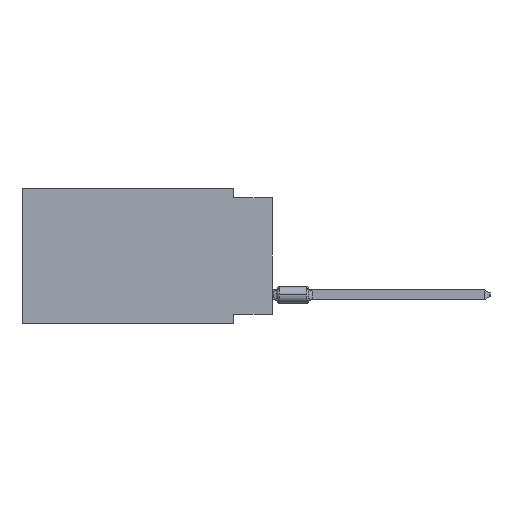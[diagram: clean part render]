
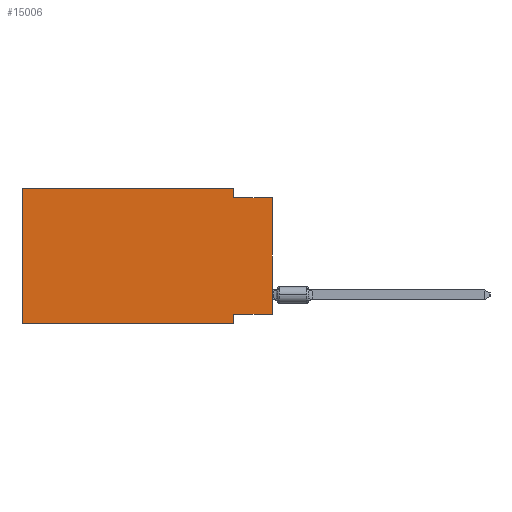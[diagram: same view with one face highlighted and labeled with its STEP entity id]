
A CAD part, left-side view. The second image highlights one B-rep face of the part: STEP entity #15006.
In plain terms, the highlighted planar face has unit normal (-1, 0, 0).
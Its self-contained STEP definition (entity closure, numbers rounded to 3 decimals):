
#209 = VERTEX_POINT ( 'NONE', #43237 ) ;
#4136 = EDGE_LOOP ( 'NONE', ( #37250, #56222, #58928, #13688, #12951, #16523, #34492, #6869 ) ) ;
#4829 = DIRECTION ( 'NONE',  ( 0., -1., 0. ) ) ;
#5136 = CARTESIAN_POINT ( 'NONE',  ( 0., 0., -0.635 ) ) ;
#6869 = ORIENTED_EDGE ( 'NONE', *, *, #29010, .F. ) ;
#7972 = LINE ( 'NONE', #22600, #20608 ) ;
#8087 = DIRECTION ( 'NONE',  ( 0., 0., -1. ) ) ;
#8434 = DIRECTION ( 'NONE',  ( 0., 0., 1. ) ) ;
#9926 = LINE ( 'NONE', #5136, #43193 ) ;
#11320 = CARTESIAN_POINT ( 'NONE',  ( 0., 16.383, 0. ) ) ;
#11420 = EDGE_CURVE ( 'NONE', #49928, #30665, #17992, .T. ) ;
#12259 = DIRECTION ( 'NONE',  ( 0., 0., -1. ) ) ;
#12860 = DIRECTION ( 'NONE',  ( 1., 0., 0. ) ) ;
#12913 = VERTEX_POINT ( 'NONE', #36321 ) ;
#12951 = ORIENTED_EDGE ( 'NONE', *, *, #53997, .F. ) ;
#13688 = ORIENTED_EDGE ( 'NONE', *, *, #23659, .F. ) ;
#15006 = ADVANCED_FACE ( 'NONE', ( #26875 ), #35800, .F. ) ;
#15818 = VERTEX_POINT ( 'NONE', #46158 ) ;
#16523 = ORIENTED_EDGE ( 'NONE', *, *, #24116, .T. ) ;
#17992 = LINE ( 'NONE', #62234, #51945 ) ;
#18377 = LINE ( 'NONE', #28557, #27778 ) ;
#19255 = VECTOR ( 'NONE', #44819, 1000. ) ;
#19465 = CARTESIAN_POINT ( 'NONE',  ( 0., 0., -8.255 ) ) ;
#20072 = CARTESIAN_POINT ( 'NONE',  ( 0., 16.383, 0. ) ) ;
#20608 = VECTOR ( 'NONE', #42022, 1000. ) ;
#22600 = CARTESIAN_POINT ( 'NONE',  ( 0., 16.383, 0. ) ) ;
#23659 = EDGE_CURVE ( 'NONE', #49332, #15818, #7972, .T. ) ;
#24116 = EDGE_CURVE ( 'NONE', #209, #12913, #18377, .T. ) ;
#24132 = VECTOR ( 'NONE', #63009, 1000. ) ;
#24517 = LINE ( 'NONE', #20072, #24132 ) ;
#26875 = FACE_OUTER_BOUND ( 'NONE', #4136, .T. ) ;
#27033 = LINE ( 'NONE', #41981, #29446 ) ;
#27778 = VECTOR ( 'NONE', #53075, 1000. ) ;
#28557 = CARTESIAN_POINT ( 'NONE',  ( 0., 16.383, -8.89 ) ) ;
#29010 = EDGE_CURVE ( 'NONE', #49928, #47721, #27033, .T. ) ;
#29446 = VECTOR ( 'NONE', #61087, 1000. ) ;
#30665 = VERTEX_POINT ( 'NONE', #57943 ) ;
#34492 = ORIENTED_EDGE ( 'NONE', *, *, #48266, .F. ) ;
#35800 = PLANE ( 'NONE',  #53589 ) ;
#36321 = CARTESIAN_POINT ( 'NONE',  ( 0., 2.54, -8.89 ) ) ;
#37250 = ORIENTED_EDGE ( 'NONE', *, *, #11420, .T. ) ;
#37402 = CARTESIAN_POINT ( 'NONE',  ( 0., 2.54, 0. ) ) ;
#41237 = LINE ( 'NONE', #37402, #59203 ) ;
#41981 = CARTESIAN_POINT ( 'NONE',  ( 0., 0., -8.255 ) ) ;
#42022 = DIRECTION ( 'NONE',  ( 0., -1., 0. ) ) ;
#43193 = VECTOR ( 'NONE', #4829, 1000. ) ;
#43237 = CARTESIAN_POINT ( 'NONE',  ( 0., 16.383, -8.89 ) ) ;
#43377 = EDGE_CURVE ( 'NONE', #49168, #30665, #9926, .T. ) ;
#44511 = LINE ( 'NONE', #49907, #19255 ) ;
#44819 = DIRECTION ( 'NONE',  ( 0., 0., -1. ) ) ;
#45372 = CARTESIAN_POINT ( 'NONE',  ( 0., 16.383, 0. ) ) ;
#45767 = EDGE_CURVE ( 'NONE', #15818, #49168, #41237, .T. ) ;
#46158 = CARTESIAN_POINT ( 'NONE',  ( 0., 2.54, 0. ) ) ;
#47721 = VERTEX_POINT ( 'NONE', #61026 ) ;
#48266 = EDGE_CURVE ( 'NONE', #47721, #12913, #44511, .T. ) ;
#49168 = VERTEX_POINT ( 'NONE', #53375 ) ;
#49332 = VERTEX_POINT ( 'NONE', #11320 ) ;
#49907 = CARTESIAN_POINT ( 'NONE',  ( 0., 2.54, -8.89 ) ) ;
#49928 = VERTEX_POINT ( 'NONE', #19465 ) ;
#51945 = VECTOR ( 'NONE', #8434, 1000. ) ;
#53075 = DIRECTION ( 'NONE',  ( 0., -1., 0. ) ) ;
#53375 = CARTESIAN_POINT ( 'NONE',  ( 0., 2.54, -0.635 ) ) ;
#53589 = AXIS2_PLACEMENT_3D ( 'NONE', #45372, #12860, #8087 ) ;
#53997 = EDGE_CURVE ( 'NONE', #209, #49332, #24517, .T. ) ;
#56222 = ORIENTED_EDGE ( 'NONE', *, *, #43377, .F. ) ;
#57943 = CARTESIAN_POINT ( 'NONE',  ( 0., 0., -0.635 ) ) ;
#58928 = ORIENTED_EDGE ( 'NONE', *, *, #45767, .F. ) ;
#59203 = VECTOR ( 'NONE', #12259, 1000. ) ;
#61026 = CARTESIAN_POINT ( 'NONE',  ( 0., 2.54, -8.255 ) ) ;
#61087 = DIRECTION ( 'NONE',  ( 0., 1., 0. ) ) ;
#62234 = CARTESIAN_POINT ( 'NONE',  ( 0., 0., 0. ) ) ;
#63009 = DIRECTION ( 'NONE',  ( 0., 0., 1. ) ) ;
